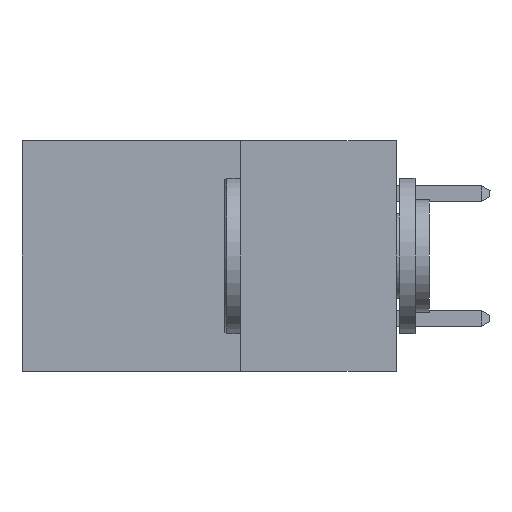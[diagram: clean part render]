
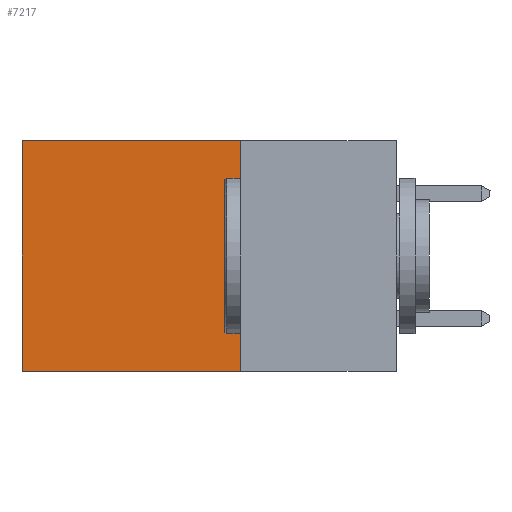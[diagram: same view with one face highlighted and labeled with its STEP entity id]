
A CAD part, left-side view. The second image highlights one B-rep face of the part: STEP entity #7217.
In plain terms, the highlighted planar face has unit normal (-1, 0, 0).
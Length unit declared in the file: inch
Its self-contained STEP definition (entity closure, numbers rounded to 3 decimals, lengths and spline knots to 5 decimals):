
#740 = DIRECTION ( 'NONE',  ( 0., 0., -1. ) ) ;
#1578 = DIRECTION ( 'NONE',  ( 0., 0., -1. ) ) ;
#2074 = DIRECTION ( 'NONE',  ( 1., 0., 0. ) ) ;
#3614 = EDGE_LOOP ( 'NONE', ( #16274, #26629, #14450, #21564 ) ) ;
#4368 = VERTEX_POINT ( 'NONE', #15683 ) ;
#4466 = LINE ( 'NONE', #22330, #9341 ) ;
#5243 = CARTESIAN_POINT ( 'NONE',  ( 0.298, 0.25, 0. ) ) ;
#5301 = CARTESIAN_POINT ( 'NONE',  ( 0.298, 0.25, -0.37 ) ) ;
#6989 = VERTEX_POINT ( 'NONE', #24244 ) ;
#7217 = ADVANCED_FACE ( 'NONE', ( #26022 ), #21929, .F. ) ;
#7926 = VECTOR ( 'NONE', #740, 39.37008 ) ;
#7977 = DIRECTION ( 'NONE',  ( 0., 0., -1. ) ) ;
#9341 = VECTOR ( 'NONE', #1578, 39.37008 ) ;
#9815 = CARTESIAN_POINT ( 'NONE',  ( 0.298, 0.25, -0.37 ) ) ;
#12053 = CARTESIAN_POINT ( 'NONE',  ( 0.298, 0.25, 0. ) ) ;
#13150 = CARTESIAN_POINT ( 'NONE',  ( 0.298, 0.6, 0. ) ) ;
#13376 = VECTOR ( 'NONE', #25822, 39.37008 ) ;
#14091 = LINE ( 'NONE', #13150, #7926 ) ;
#14151 = VECTOR ( 'NONE', #21750, 39.37008 ) ;
#14200 = VERTEX_POINT ( 'NONE', #9815 ) ;
#14450 = ORIENTED_EDGE ( 'NONE', *, *, #25961, .F. ) ;
#15683 = CARTESIAN_POINT ( 'NONE',  ( 0.298, 0.25, 0. ) ) ;
#16274 = ORIENTED_EDGE ( 'NONE', *, *, #19582, .T. ) ;
#16288 = AXIS2_PLACEMENT_3D ( 'NONE', #12053, #2074, #7977 ) ;
#16311 = CARTESIAN_POINT ( 'NONE',  ( 0.298, 0.6, 0. ) ) ;
#18838 = LINE ( 'NONE', #5301, #13376 ) ;
#19116 = EDGE_CURVE ( 'NONE', #14200, #6989, #18838, .T. ) ;
#19582 = EDGE_CURVE ( 'NONE', #25388, #6989, #14091, .T. ) ;
#19601 = LINE ( 'NONE', #5243, #14151 ) ;
#21564 = ORIENTED_EDGE ( 'NONE', *, *, #26342, .T. ) ;
#21750 = DIRECTION ( 'NONE',  ( 0., 1., 0. ) ) ;
#21929 = PLANE ( 'NONE',  #16288 ) ;
#22330 = CARTESIAN_POINT ( 'NONE',  ( 0.298, 0.25, 0. ) ) ;
#24244 = CARTESIAN_POINT ( 'NONE',  ( 0.298, 0.6, -0.37 ) ) ;
#25388 = VERTEX_POINT ( 'NONE', #16311 ) ;
#25822 = DIRECTION ( 'NONE',  ( 0., 1., 0. ) ) ;
#25961 = EDGE_CURVE ( 'NONE', #4368, #14200, #4466, .T. ) ;
#26022 = FACE_OUTER_BOUND ( 'NONE', #3614, .T. ) ;
#26342 = EDGE_CURVE ( 'NONE', #4368, #25388, #19601, .T. ) ;
#26629 = ORIENTED_EDGE ( 'NONE', *, *, #19116, .F. ) ;
